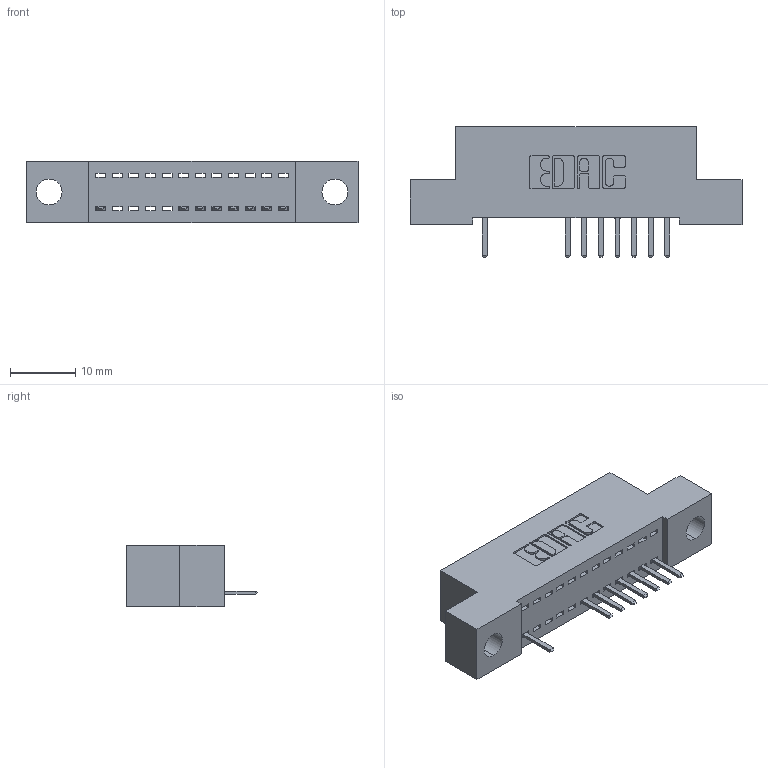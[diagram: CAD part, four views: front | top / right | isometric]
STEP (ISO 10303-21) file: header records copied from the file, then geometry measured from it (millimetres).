
FILE_DESCRIPTION (( 'STEP AP203' ), '1' );
FILE_NAME ('392-012-520-104.STEP', '2018-08-14T21:37:33', ( '' ), ( '' ), 'SwSTEP 2.0', 'SolidWorks 2016', '' );
FILE_SCHEMA (( 'CONFIG_CONTROL_DESIGN' ));
Length unit declared in the file: inch
Products named in the file (3): 342 Part_.156 TH; 345-292-001_345-293-120; 392-012-520-104
Assembly tree (9 placements, depth 2):
  392-012-520-104
    342 Part_.156 TH
    345-292-001_345-293-120  x8
Bounding box: 50.8 x 20.02 x 9.4 mm (x, y, z)
Volume: 4187.9 mm3; surface area: 5097.7 mm2
Topology: 9 solids, 9 shells, 654 faces, 1939 edges, 1270 vertices
Faces by surface type: plane 466, cylinder 188
Entity records: 11073 total; most frequent: CARTESIAN_POINT 1950, ORIENTED_EDGE 1890, DIRECTION 1689, EDGE_CURVE 945, VECTOR 813, LINE 813, VERTEX_POINT 626, AXIS2_PLACEMENT_3D 438
